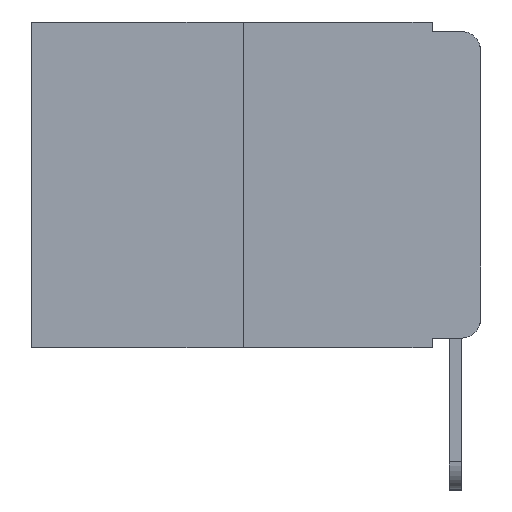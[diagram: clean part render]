
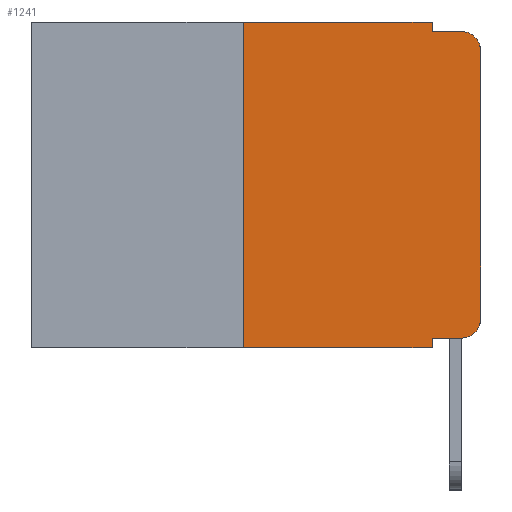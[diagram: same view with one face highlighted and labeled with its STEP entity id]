
A CAD part, left-side view. The second image highlights one B-rep face of the part: STEP entity #1241.
In plain terms, the highlighted planar face has unit normal (-1, 0, 0).
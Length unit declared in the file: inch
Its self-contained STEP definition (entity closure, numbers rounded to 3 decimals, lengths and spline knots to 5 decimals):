
#6 = EDGE_CURVE ( 'NONE', #8336, #12677, #17546, .T. ) ;
#404 = ORIENTED_EDGE ( 'NONE', *, *, #3964, .F. ) ;
#817 = CARTESIAN_POINT ( 'NONE',  ( 0., 0.25, -0.343 ) ) ;
#990 = VERTEX_POINT ( 'NONE', #817 ) ;
#1241 = ADVANCED_FACE ( 'NONE', ( #2980 ), #3441, .F. ) ;
#1243 = CARTESIAN_POINT ( 'NONE',  ( 0., 0., 0. ) ) ;
#1771 = VERTEX_POINT ( 'NONE', #10816 ) ;
#2328 = CARTESIAN_POINT ( 'NONE',  ( 0., 0.02, -0.333 ) ) ;
#2402 = VERTEX_POINT ( 'NONE', #17374 ) ;
#2664 = CARTESIAN_POINT ( 'NONE',  ( 0., 0.051, 0. ) ) ;
#2689 = ORIENTED_EDGE ( 'NONE', *, *, #3796, .T. ) ;
#2698 = VECTOR ( 'NONE', #7854, 39.37008 ) ;
#2824 = VECTOR ( 'NONE', #14238, 39.37008 ) ;
#2980 = FACE_OUTER_BOUND ( 'NONE', #17621, .T. ) ;
#3441 = PLANE ( 'NONE',  #16628 ) ;
#3722 = LINE ( 'NONE', #17400, #4570 ) ;
#3794 = VERTEX_POINT ( 'NONE', #5084 ) ;
#3796 = EDGE_CURVE ( 'NONE', #6417, #3794, #10230, .T. ) ;
#3964 = EDGE_CURVE ( 'NONE', #1771, #3794, #3722, .T. ) ;
#4210 = EDGE_CURVE ( 'NONE', #990, #15738, #19322, .T. ) ;
#4570 = VECTOR ( 'NONE', #20448, 39.37008 ) ;
#4706 = ORIENTED_EDGE ( 'NONE', *, *, #17239, .F. ) ;
#4717 = VECTOR ( 'NONE', #19073, 39.37008 ) ;
#5025 = EDGE_CURVE ( 'NONE', #2402, #7191, #20662, .T. ) ;
#5084 = CARTESIAN_POINT ( 'NONE',  ( 0., 0.02, -0.01 ) ) ;
#5277 = CARTESIAN_POINT ( 'NONE',  ( 0., 0.473, 0. ) ) ;
#5404 = ORIENTED_EDGE ( 'NONE', *, *, #10455, .T. ) ;
#5741 = ORIENTED_EDGE ( 'NONE', *, *, #4210, .T. ) ;
#5830 = DIRECTION ( 'NONE',  ( -1., 0., 0. ) ) ;
#6016 = VECTOR ( 'NONE', #9344, 39.37008 ) ;
#6291 = CARTESIAN_POINT ( 'NONE',  ( 0., 0., -0.313 ) ) ;
#6417 = VERTEX_POINT ( 'NONE', #15278 ) ;
#6530 = CARTESIAN_POINT ( 'NONE',  ( 0., 0.051, 0. ) ) ;
#6592 = ORIENTED_EDGE ( 'NONE', *, *, #13145, .F. ) ;
#6811 = DIRECTION ( 'NONE',  ( -1., 0., 0. ) ) ;
#7191 = VERTEX_POINT ( 'NONE', #6530 ) ;
#7540 = CARTESIAN_POINT ( 'NONE',  ( 0., 0.051, -0.343 ) ) ;
#7854 = DIRECTION ( 'NONE',  ( 0., 0., -1. ) ) ;
#8336 = VERTEX_POINT ( 'NONE', #2328 ) ;
#8779 = CARTESIAN_POINT ( 'NONE',  ( 0., 0.25, 0. ) ) ;
#9329 = CARTESIAN_POINT ( 'NONE',  ( 0., 0.02, -0.313 ) ) ;
#9344 = DIRECTION ( 'NONE',  ( 0., -1., 0. ) ) ;
#9817 = LINE ( 'NONE', #2664, #4717 ) ;
#10189 = AXIS2_PLACEMENT_3D ( 'NONE', #9329, #5830, #11129 ) ;
#10203 = VECTOR ( 'NONE', #15867, 39.37008 ) ;
#10230 = CIRCLE ( 'NONE', #13284, 0.02 ) ;
#10278 = DIRECTION ( 'NONE',  ( 0., 0., -1. ) ) ;
#10455 = EDGE_CURVE ( 'NONE', #12677, #6417, #16486, .T. ) ;
#10478 = DIRECTION ( 'NONE',  ( 1., 0., 0. ) ) ;
#10816 = CARTESIAN_POINT ( 'NONE',  ( 0., 0.051, -0.01 ) ) ;
#10835 = LINE ( 'NONE', #20121, #6016 ) ;
#11129 = DIRECTION ( 'NONE',  ( 0., 0., -1. ) ) ;
#11321 = CARTESIAN_POINT ( 'NONE',  ( 0., 0.051, 0. ) ) ;
#11887 = VECTOR ( 'NONE', #23142, 39.37008 ) ;
#12356 = LINE ( 'NONE', #11321, #2698 ) ;
#12468 = DIRECTION ( 'NONE',  ( 0., -1., 0. ) ) ;
#12477 = LINE ( 'NONE', #8779, #2824 ) ;
#12677 = VERTEX_POINT ( 'NONE', #6291 ) ;
#13145 = EDGE_CURVE ( 'NONE', #22365, #15738, #12356, .T. ) ;
#13284 = AXIS2_PLACEMENT_3D ( 'NONE', #17694, #6811, #10278 ) ;
#13341 = VECTOR ( 'NONE', #12468, 39.37008 ) ;
#13541 = CARTESIAN_POINT ( 'NONE',  ( 0., 0.051, -0.333 ) ) ;
#14238 = DIRECTION ( 'NONE',  ( 0., 0., 1. ) ) ;
#15278 = CARTESIAN_POINT ( 'NONE',  ( 0., 0., -0.03 ) ) ;
#15406 = ORIENTED_EDGE ( 'NONE', *, *, #5025, .F. ) ;
#15478 = EDGE_CURVE ( 'NONE', #22365, #8336, #10835, .T. ) ;
#15738 = VERTEX_POINT ( 'NONE', #7540 ) ;
#15867 = DIRECTION ( 'NONE',  ( 0., 0., 1. ) ) ;
#15884 = ORIENTED_EDGE ( 'NONE', *, *, #22920, .F. ) ;
#16098 = ORIENTED_EDGE ( 'NONE', *, *, #6, .T. ) ;
#16486 = LINE ( 'NONE', #1243, #10203 ) ;
#16628 = AXIS2_PLACEMENT_3D ( 'NONE', #5277, #10478, #19841 ) ;
#17239 = EDGE_CURVE ( 'NONE', #990, #2402, #12477, .T. ) ;
#17374 = CARTESIAN_POINT ( 'NONE',  ( 0., 0.25, 0. ) ) ;
#17400 = CARTESIAN_POINT ( 'NONE',  ( 0., 0.051, -0.01 ) ) ;
#17546 = CIRCLE ( 'NONE', #10189, 0.02 ) ;
#17621 = EDGE_LOOP ( 'NONE', ( #5404, #2689, #404, #15884, #15406, #4706, #5741, #6592, #22282, #16098 ) ) ;
#17694 = CARTESIAN_POINT ( 'NONE',  ( 0., 0.02, -0.03 ) ) ;
#19073 = DIRECTION ( 'NONE',  ( 0., 0., -1. ) ) ;
#19322 = LINE ( 'NONE', #21566, #13341 ) ;
#19841 = DIRECTION ( 'NONE',  ( 0., 0., -1. ) ) ;
#19910 = CARTESIAN_POINT ( 'NONE',  ( 0., 0.473, 0. ) ) ;
#20121 = CARTESIAN_POINT ( 'NONE',  ( 0., 0.051, -0.333 ) ) ;
#20448 = DIRECTION ( 'NONE',  ( 0., -1., 0. ) ) ;
#20662 = LINE ( 'NONE', #19910, #11887 ) ;
#21566 = CARTESIAN_POINT ( 'NONE',  ( 0., 0.473, -0.343 ) ) ;
#22282 = ORIENTED_EDGE ( 'NONE', *, *, #15478, .T. ) ;
#22365 = VERTEX_POINT ( 'NONE', #13541 ) ;
#22920 = EDGE_CURVE ( 'NONE', #7191, #1771, #9817, .T. ) ;
#23142 = DIRECTION ( 'NONE',  ( 0., -1., 0. ) ) ;
